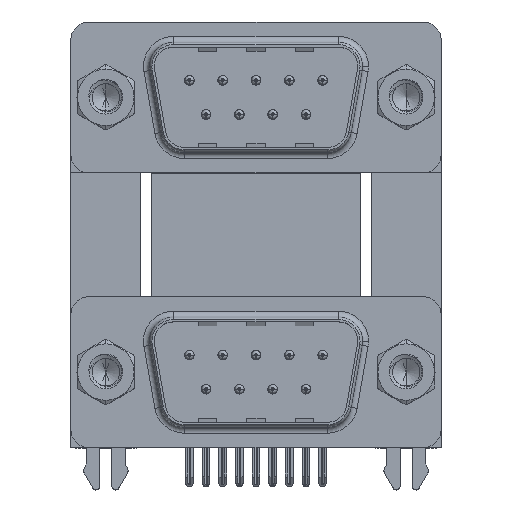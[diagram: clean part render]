
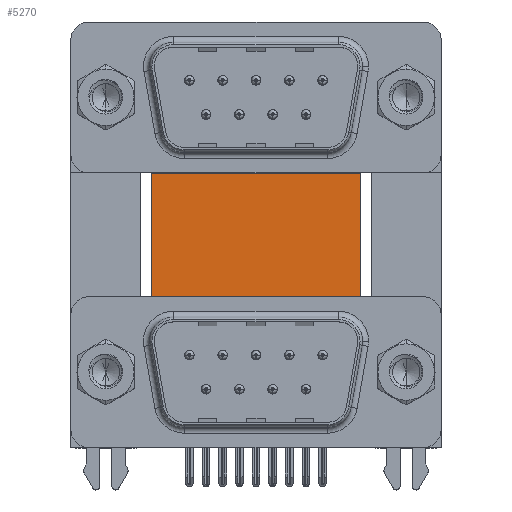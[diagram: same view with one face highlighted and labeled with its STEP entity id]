
A CAD part, top view. The second image highlights one B-rep face of the part: STEP entity #5270.
In plain terms, the highlighted planar face has unit normal (0, 0, 1).
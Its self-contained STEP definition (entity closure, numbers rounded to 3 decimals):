
#1326 = LINE ( 'NONE', #11414, #31799 ) ;
#2557 = DIRECTION ( 'NONE',  ( 0., 0., -1. ) ) ;
#3177 = AXIS2_PLACEMENT_3D ( 'NONE', #5412, #2557, #8267 ) ;
#3599 = CARTESIAN_POINT ( 'NONE',  ( 21.2, -0.735, -12. ) ) ;
#3902 = EDGE_CURVE ( 'NONE', #9458, #27949, #29305, .T. ) ;
#4067 = DIRECTION ( 'NONE',  ( 0., -1., 0. ) ) ;
#4194 = EDGE_CURVE ( 'NONE', #6220, #19799, #14759, .T. ) ;
#4238 = LINE ( 'NONE', #7409, #23257 ) ;
#5270 = ADVANCED_FACE ( 'NONE', ( #33147 ), #15672, .F. ) ;
#5412 = CARTESIAN_POINT ( 'NONE',  ( 3.79, 16.585, -12. ) ) ;
#6215 = LINE ( 'NONE', #31606, #32203 ) ;
#6220 = VERTEX_POINT ( 'NONE', #30841 ) ;
#6423 = CARTESIAN_POINT ( 'NONE',  ( 22.09, -4.635, -12. ) ) ;
#6516 = ORIENTED_EDGE ( 'NONE', *, *, #25694, .T. ) ;
#6804 = EDGE_CURVE ( 'NONE', #21329, #19799, #13826, .T. ) ;
#7068 = CARTESIAN_POINT ( 'NONE',  ( 3.79, 16.585, -12. ) ) ;
#7356 = CARTESIAN_POINT ( 'NONE',  ( 22.59, -4.635, -12. ) ) ;
#7409 = CARTESIAN_POINT ( 'NONE',  ( 3.79, -3.735, -12. ) ) ;
#7862 = DIRECTION ( 'NONE',  ( -0.336, -0.942, 0. ) ) ;
#8086 = VERTEX_POINT ( 'NONE', #32953 ) ;
#8193 = CARTESIAN_POINT ( 'NONE',  ( 2.4, -4.635, -12. ) ) ;
#8267 = DIRECTION ( 'NONE',  ( -1., 0., 0. ) ) ;
#8767 = ORIENTED_EDGE ( 'NONE', *, *, #10754, .T. ) ;
#8909 = DIRECTION ( 'NONE',  ( 0., 1., 0. ) ) ;
#9458 = VERTEX_POINT ( 'NONE', #11450 ) ;
#9894 = VECTOR ( 'NONE', #24161, 1000. ) ;
#10068 = ORIENTED_EDGE ( 'NONE', *, *, #18540, .T. ) ;
#10670 = ORIENTED_EDGE ( 'NONE', *, *, #21849, .T. ) ;
#10754 = EDGE_CURVE ( 'NONE', #8086, #21322, #1326, .T. ) ;
#10885 = CARTESIAN_POINT ( 'NONE',  ( 3.79, 16.585, -12. ) ) ;
#11414 = CARTESIAN_POINT ( 'NONE',  ( 2.9, -3.735, -12. ) ) ;
#11450 = CARTESIAN_POINT ( 'NONE',  ( 22.09, -3.735, -12. ) ) ;
#11588 = EDGE_CURVE ( 'NONE', #21322, #9458, #4238, .T. ) ;
#11692 = ORIENTED_EDGE ( 'NONE', *, *, #11588, .T. ) ;
#11968 = VECTOR ( 'NONE', #31534, 1000. ) ;
#12228 = ORIENTED_EDGE ( 'NONE', *, *, #3902, .T. ) ;
#13258 = VECTOR ( 'NONE', #7862, 1000. ) ;
#13826 = LINE ( 'NONE', #32289, #28499 ) ;
#13994 = CARTESIAN_POINT ( 'NONE',  ( 2.9, -3.735, -12. ) ) ;
#14577 = EDGE_CURVE ( 'NONE', #25199, #21329, #18944, .T. ) ;
#14759 = LINE ( 'NONE', #7356, #14948 ) ;
#14948 = VECTOR ( 'NONE', #30047, 1000. ) ;
#15672 = PLANE ( 'NONE',  #3177 ) ;
#15805 = LINE ( 'NONE', #21194, #22317 ) ;
#16148 = DIRECTION ( 'NONE',  ( 1., 0., 0. ) ) ;
#16488 = DIRECTION ( 'NONE',  ( 1., 0., 0. ) ) ;
#18540 = EDGE_CURVE ( 'NONE', #25199, #21260, #28513, .T. ) ;
#18944 = LINE ( 'NONE', #10885, #9894 ) ;
#19466 = EDGE_LOOP ( 'NONE', ( #11692, #12228, #10670, #22236, #30115, #32022, #10068, #6516, #22268, #8767 ) ) ;
#19799 = VERTEX_POINT ( 'NONE', #3599 ) ;
#20233 = CARTESIAN_POINT ( 'NONE',  ( 3.79, -0.735, -12. ) ) ;
#20881 = VECTOR ( 'NONE', #21753, 1000. ) ;
#21194 = CARTESIAN_POINT ( 'NONE',  ( 22.09, -4.635, -12. ) ) ;
#21260 = VERTEX_POINT ( 'NONE', #20233 ) ;
#21322 = VERTEX_POINT ( 'NONE', #13994 ) ;
#21329 = VERTEX_POINT ( 'NONE', #23913 ) ;
#21753 = DIRECTION ( 'NONE',  ( 0., -1., 0. ) ) ;
#21849 = EDGE_CURVE ( 'NONE', #27949, #6220, #15805, .T. ) ;
#22049 = VERTEX_POINT ( 'NONE', #24705 ) ;
#22236 = ORIENTED_EDGE ( 'NONE', *, *, #4194, .T. ) ;
#22268 = ORIENTED_EDGE ( 'NONE', *, *, #29050, .T. ) ;
#22317 = VECTOR ( 'NONE', #16148, 1000. ) ;
#23257 = VECTOR ( 'NONE', #30602, 1000. ) ;
#23913 = CARTESIAN_POINT ( 'NONE',  ( 21.2, 16.585, -12. ) ) ;
#24161 = DIRECTION ( 'NONE',  ( 1., 0., 0. ) ) ;
#24607 = CARTESIAN_POINT ( 'NONE',  ( 22.09, -3.735, -12. ) ) ;
#24705 = CARTESIAN_POINT ( 'NONE',  ( 2.4, -4.635, -12. ) ) ;
#25199 = VERTEX_POINT ( 'NONE', #7068 ) ;
#25694 = EDGE_CURVE ( 'NONE', #21260, #22049, #31052, .T. ) ;
#27949 = VERTEX_POINT ( 'NONE', #6423 ) ;
#28499 = VECTOR ( 'NONE', #4067, 1000. ) ;
#28513 = LINE ( 'NONE', #29022, #11968 ) ;
#29022 = CARTESIAN_POINT ( 'NONE',  ( 3.79, 16.585, -12. ) ) ;
#29050 = EDGE_CURVE ( 'NONE', #22049, #8086, #6215, .T. ) ;
#29305 = LINE ( 'NONE', #24607, #20881 ) ;
#30047 = DIRECTION ( 'NONE',  ( -0.336, 0.942, 0. ) ) ;
#30115 = ORIENTED_EDGE ( 'NONE', *, *, #6804, .F. ) ;
#30602 = DIRECTION ( 'NONE',  ( 1., 0., 0. ) ) ;
#30841 = CARTESIAN_POINT ( 'NONE',  ( 22.59, -4.635, -12. ) ) ;
#31052 = LINE ( 'NONE', #8193, #13258 ) ;
#31534 = DIRECTION ( 'NONE',  ( 0., -1., 0. ) ) ;
#31606 = CARTESIAN_POINT ( 'NONE',  ( 2.9, -4.635, -12. ) ) ;
#31799 = VECTOR ( 'NONE', #8909, 1000. ) ;
#32022 = ORIENTED_EDGE ( 'NONE', *, *, #14577, .F. ) ;
#32203 = VECTOR ( 'NONE', #16488, 1000. ) ;
#32289 = CARTESIAN_POINT ( 'NONE',  ( 21.2, 16.585, -12. ) ) ;
#32953 = CARTESIAN_POINT ( 'NONE',  ( 2.9, -4.635, -12. ) ) ;
#33147 = FACE_OUTER_BOUND ( 'NONE', #19466, .T. ) ;
